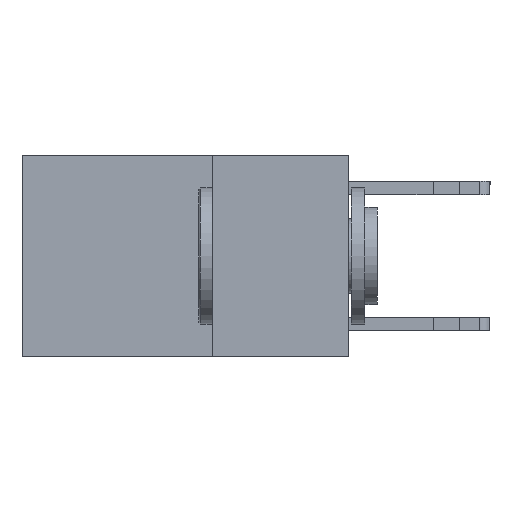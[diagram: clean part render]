
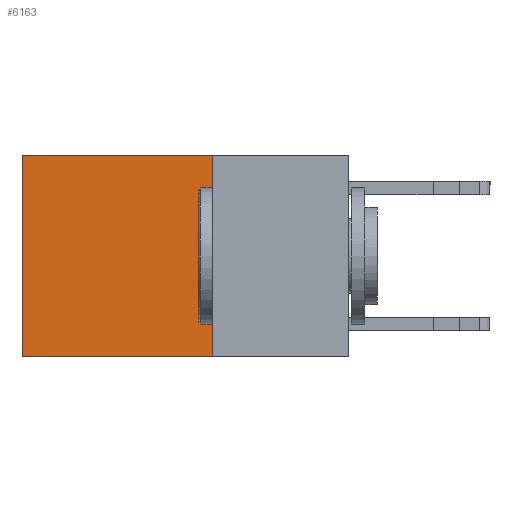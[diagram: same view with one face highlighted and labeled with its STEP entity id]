
A CAD part, left-side view. The second image highlights one B-rep face of the part: STEP entity #6163.
In plain terms, the highlighted planar face has unit normal (-1, 0, 0).
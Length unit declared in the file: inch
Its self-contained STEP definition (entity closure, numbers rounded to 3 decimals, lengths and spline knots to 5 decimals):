
#451 = EDGE_CURVE ( 'NONE', #12823, #12885, #10254, .T. ) ;
#1111 = VECTOR ( 'NONE', #2444, 39.37008 ) ;
#1531 = EDGE_CURVE ( 'NONE', #12885, #4495, #7733, .T. ) ;
#1960 = CARTESIAN_POINT ( 'NONE',  ( 0.2625, 0.25, 0. ) ) ;
#2444 = DIRECTION ( 'NONE',  ( 0., 0., -1. ) ) ;
#2540 = DIRECTION ( 'NONE',  ( 0., 1., 0. ) ) ;
#2874 = CARTESIAN_POINT ( 'NONE',  ( 0.2625, 0.6, 0. ) ) ;
#3865 = CARTESIAN_POINT ( 'NONE',  ( 0.2625, 0.25, 0. ) ) ;
#4157 = VERTEX_POINT ( 'NONE', #2874 ) ;
#4353 = DIRECTION ( 'NONE',  ( 0., 0., -1. ) ) ;
#4495 = VERTEX_POINT ( 'NONE', #12801 ) ;
#4876 = LINE ( 'NONE', #12078, #5535 ) ;
#5378 = FACE_OUTER_BOUND ( 'NONE', #13026, .T. ) ;
#5464 = EDGE_CURVE ( 'NONE', #12823, #4157, #4876, .T. ) ;
#5535 = VECTOR ( 'NONE', #2540, 39.37008 ) ;
#5991 = AXIS2_PLACEMENT_3D ( 'NONE', #7651, #11760, #4353 ) ;
#6163 = ADVANCED_FACE ( 'NONE', ( #5378 ), #12851, .F. ) ;
#6827 = CARTESIAN_POINT ( 'NONE',  ( 0.2625, 0.6, 0. ) ) ;
#7601 = VECTOR ( 'NONE', #10315, 39.37008 ) ;
#7651 = CARTESIAN_POINT ( 'NONE',  ( 0.2625, 0.25, 0. ) ) ;
#7733 = LINE ( 'NONE', #9718, #7836 ) ;
#7832 = EDGE_CURVE ( 'NONE', #4157, #4495, #7858, .T. ) ;
#7836 = VECTOR ( 'NONE', #12997, 39.37008 ) ;
#7858 = LINE ( 'NONE', #6827, #1111 ) ;
#8395 = ORIENTED_EDGE ( 'NONE', *, *, #451, .F. ) ;
#8983 = ORIENTED_EDGE ( 'NONE', *, *, #7832, .T. ) ;
#9119 = ORIENTED_EDGE ( 'NONE', *, *, #1531, .F. ) ;
#9718 = CARTESIAN_POINT ( 'NONE',  ( 0.2625, 0.25, -0.37 ) ) ;
#10254 = LINE ( 'NONE', #1960, #7601 ) ;
#10315 = DIRECTION ( 'NONE',  ( 0., 0., -1. ) ) ;
#11150 = ORIENTED_EDGE ( 'NONE', *, *, #5464, .T. ) ;
#11760 = DIRECTION ( 'NONE',  ( 1., 0., 0. ) ) ;
#12078 = CARTESIAN_POINT ( 'NONE',  ( 0.2625, 0.25, 0. ) ) ;
#12515 = CARTESIAN_POINT ( 'NONE',  ( 0.2625, 0.25, -0.37 ) ) ;
#12801 = CARTESIAN_POINT ( 'NONE',  ( 0.2625, 0.6, -0.37 ) ) ;
#12823 = VERTEX_POINT ( 'NONE', #3865 ) ;
#12851 = PLANE ( 'NONE',  #5991 ) ;
#12885 = VERTEX_POINT ( 'NONE', #12515 ) ;
#12997 = DIRECTION ( 'NONE',  ( 0., 1., 0. ) ) ;
#13026 = EDGE_LOOP ( 'NONE', ( #8983, #9119, #8395, #11150 ) ) ;
